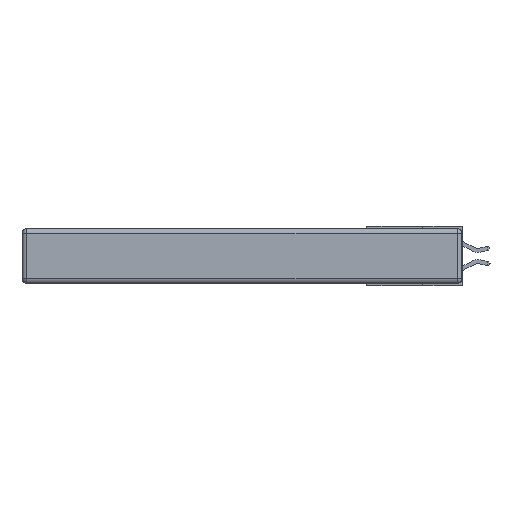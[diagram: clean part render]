
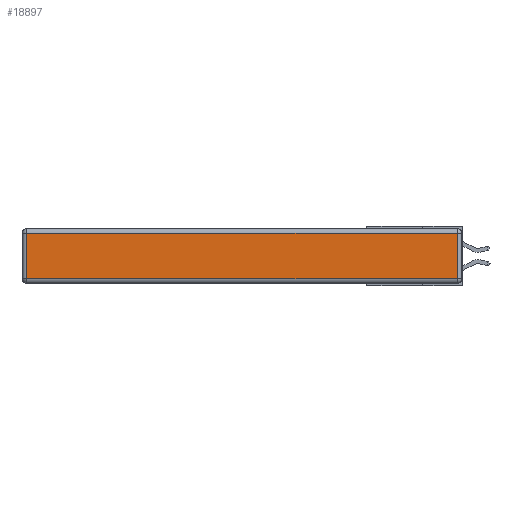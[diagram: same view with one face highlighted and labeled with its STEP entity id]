
A CAD part, left-side view. The second image highlights one B-rep face of the part: STEP entity #18897.
In plain terms, the highlighted planar face has unit normal (-1, 0, 0).
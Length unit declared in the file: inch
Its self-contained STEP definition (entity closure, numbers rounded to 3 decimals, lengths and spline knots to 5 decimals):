
#660 = ORIENTED_EDGE ( 'NONE', *, *, #9068, .T. ) ;
#5146 = EDGE_LOOP ( 'NONE', ( #26573, #32270, #660, #17609 ) ) ;
#5524 = CARTESIAN_POINT ( 'NONE',  ( 0., 0., -0.313 ) ) ;
#7859 = AXIS2_PLACEMENT_3D ( 'NONE', #33300, #13734, #16342 ) ;
#8449 = DIRECTION ( 'NONE',  ( 0., 1., 0. ) ) ;
#8942 = LINE ( 'NONE', #30262, #31695 ) ;
#9068 = EDGE_CURVE ( 'NONE', #20860, #9499, #8942, .T. ) ;
#9213 = CARTESIAN_POINT ( 'NONE',  ( 0., 2.72, -0.313 ) ) ;
#9363 = CARTESIAN_POINT ( 'NONE',  ( 0., 0.03, -0.03 ) ) ;
#9499 = VERTEX_POINT ( 'NONE', #22115 ) ;
#13734 = DIRECTION ( 'NONE',  ( -1., 0., 0. ) ) ;
#14511 = CARTESIAN_POINT ( 'NONE',  ( 0., 0.03, -0.313 ) ) ;
#14555 = DIRECTION ( 'NONE',  ( 0., 0., 1. ) ) ;
#16342 = DIRECTION ( 'NONE',  ( 0., 0., 1. ) ) ;
#17609 = ORIENTED_EDGE ( 'NONE', *, *, #29750, .T. ) ;
#18897 = ADVANCED_FACE ( 'NONE', ( #31217 ), #27400, .T. ) ;
#19916 = CARTESIAN_POINT ( 'NONE',  ( 0., 0.03, -0.343 ) ) ;
#19989 = EDGE_CURVE ( 'NONE', #27677, #34678, #28186, .T. ) ;
#20140 = LINE ( 'NONE', #30180, #23141 ) ;
#20860 = VERTEX_POINT ( 'NONE', #9363 ) ;
#22115 = CARTESIAN_POINT ( 'NONE',  ( 0., 2.72, -0.03 ) ) ;
#22836 = VECTOR ( 'NONE', #14555, 39.37008 ) ;
#23141 = VECTOR ( 'NONE', #30552, 39.37008 ) ;
#26573 = ORIENTED_EDGE ( 'NONE', *, *, #19989, .T. ) ;
#27085 = DIRECTION ( 'NONE',  ( 0., -1., 0. ) ) ;
#27118 = LINE ( 'NONE', #19916, #22836 ) ;
#27400 = PLANE ( 'NONE',  #7859 ) ;
#27677 = VERTEX_POINT ( 'NONE', #9213 ) ;
#28186 = LINE ( 'NONE', #5524, #33354 ) ;
#28557 = EDGE_CURVE ( 'NONE', #34678, #20860, #27118, .T. ) ;
#29750 = EDGE_CURVE ( 'NONE', #9499, #27677, #20140, .T. ) ;
#30180 = CARTESIAN_POINT ( 'NONE',  ( 0., 2.72, -0.343 ) ) ;
#30262 = CARTESIAN_POINT ( 'NONE',  ( 0., 2.75, -0.03 ) ) ;
#30552 = DIRECTION ( 'NONE',  ( 0., 0., -1. ) ) ;
#31217 = FACE_OUTER_BOUND ( 'NONE', #5146, .T. ) ;
#31695 = VECTOR ( 'NONE', #8449, 39.37008 ) ;
#32270 = ORIENTED_EDGE ( 'NONE', *, *, #28557, .T. ) ;
#33300 = CARTESIAN_POINT ( 'NONE',  ( 0., 0., -0.343 ) ) ;
#33354 = VECTOR ( 'NONE', #27085, 39.37008 ) ;
#34678 = VERTEX_POINT ( 'NONE', #14511 ) ;
